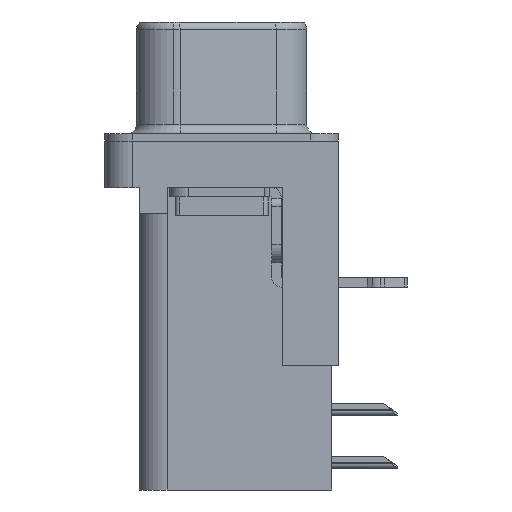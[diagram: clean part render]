
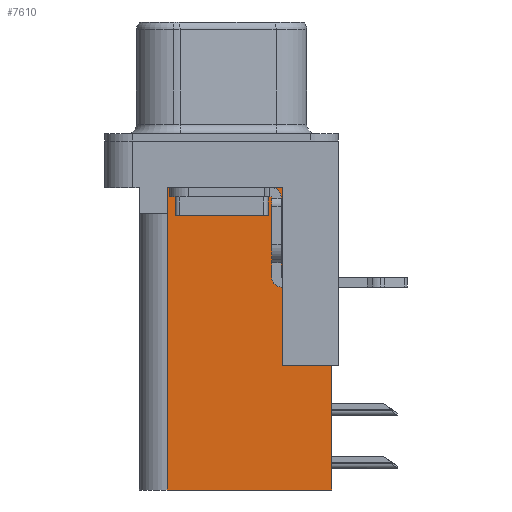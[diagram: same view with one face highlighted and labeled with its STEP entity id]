
A CAD part, left-side view. The second image highlights one B-rep face of the part: STEP entity #7610.
In plain terms, the highlighted planar face has unit normal (-1, 0, 0).
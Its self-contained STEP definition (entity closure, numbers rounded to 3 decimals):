
#11 = CARTESIAN_POINT ( 'NONE',  ( 3.7, 0., -3.9 ) ) ;
#113 = AXIS2_PLACEMENT_3D ( 'NONE', #18830, #20484, #10720 ) ;
#139 = ORIENTED_EDGE ( 'NONE', *, *, #1544, .F. ) ;
#340 = VERTEX_POINT ( 'NONE', #14604 ) ;
#858 = VECTOR ( 'NONE', #15821, 1000. ) ;
#1153 = CARTESIAN_POINT ( 'NONE',  ( 3.7, -5.925, -18.76 ) ) ;
#1157 = CARTESIAN_POINT ( 'NONE',  ( 3.7, -5.925, -2. ) ) ;
#1219 = VERTEX_POINT ( 'NONE', #19559 ) ;
#1384 = LINE ( 'NONE', #1157, #19120 ) ;
#1544 = EDGE_CURVE ( 'NONE', #19565, #340, #17263, .T. ) ;
#1650 = DIRECTION ( 'NONE',  ( 0., 1., 0. ) ) ;
#2764 = DIRECTION ( 'NONE',  ( 0., 1., 0. ) ) ;
#3130 = CARTESIAN_POINT ( 'NONE',  ( 3.7, 2.895, -3.9 ) ) ;
#3639 = VECTOR ( 'NONE', #14494, 1000. ) ;
#3640 = VECTOR ( 'NONE', #3860, 1000. ) ;
#3668 = VERTEX_POINT ( 'NONE', #13161 ) ;
#3860 = DIRECTION ( 'NONE',  ( 0., 0., -1. ) ) ;
#4145 = VECTOR ( 'NONE', #1650, 1000. ) ;
#4153 = LINE ( 'NONE', #9622, #3639 ) ;
#4337 = VECTOR ( 'NONE', #2764, 1000. ) ;
#4493 = CARTESIAN_POINT ( 'NONE',  ( 3.7, -3.295, -2.5 ) ) ;
#5072 = CARTESIAN_POINT ( 'NONE',  ( 3.7, -5.925, -12.05 ) ) ;
#5366 = VERTEX_POINT ( 'NONE', #12858 ) ;
#5698 = VECTOR ( 'NONE', #15440, 1000. ) ;
#5720 = CARTESIAN_POINT ( 'NONE',  ( 3.7, -6.295, -12.05 ) ) ;
#5996 = CARTESIAN_POINT ( 'NONE',  ( 3.7, 2.925, -3.9 ) ) ;
#6307 = CARTESIAN_POINT ( 'NONE',  ( 3.7, -3.295, -18.76 ) ) ;
#6453 = EDGE_CURVE ( 'NONE', #14682, #19565, #1384, .T. ) ;
#6469 = EDGE_CURVE ( 'NONE', #5366, #1219, #17591, .T. ) ;
#6538 = EDGE_CURVE ( 'NONE', #8450, #12078, #12741, .T. ) ;
#6655 = ORIENTED_EDGE ( 'NONE', *, *, #11893, .T. ) ;
#7006 = ORIENTED_EDGE ( 'NONE', *, *, #18163, .F. ) ;
#7356 = ORIENTED_EDGE ( 'NONE', *, *, #11287, .T. ) ;
#7496 = PLANE ( 'NONE',  #113 ) ;
#7610 = ADVANCED_FACE ( 'NONE', ( #12400 ), #7496, .F. ) ;
#8450 = VERTEX_POINT ( 'NONE', #3130 ) ;
#8936 = ORIENTED_EDGE ( 'NONE', *, *, #6538, .T. ) ;
#9622 = CARTESIAN_POINT ( 'NONE',  ( 3.7, -3.295, -18.76 ) ) ;
#9951 = ORIENTED_EDGE ( 'NONE', *, *, #6453, .F. ) ;
#9954 = ORIENTED_EDGE ( 'NONE', *, *, #6469, .T. ) ;
#10021 = LINE ( 'NONE', #5720, #5698 ) ;
#10720 = DIRECTION ( 'NONE',  ( 0., 1., 0. ) ) ;
#10790 = ORIENTED_EDGE ( 'NONE', *, *, #15153, .T. ) ;
#11287 = EDGE_CURVE ( 'NONE', #14682, #3668, #10021, .T. ) ;
#11893 = EDGE_CURVE ( 'NONE', #1219, #8450, #12241, .T. ) ;
#11927 = CARTESIAN_POINT ( 'NONE',  ( 3.7, 2.925, -18.76 ) ) ;
#12078 = VERTEX_POINT ( 'NONE', #5996 ) ;
#12241 = LINE ( 'NONE', #15208, #3640 ) ;
#12400 = FACE_OUTER_BOUND ( 'NONE', #18808, .T. ) ;
#12454 = DIRECTION ( 'NONE',  ( 0., 0., -1. ) ) ;
#12741 = LINE ( 'NONE', #11, #4145 ) ;
#12858 = CARTESIAN_POINT ( 'NONE',  ( 3.7, -3.295, -2.5 ) ) ;
#13161 = CARTESIAN_POINT ( 'NONE',  ( 3.7, -3.295, -12.05 ) ) ;
#14494 = DIRECTION ( 'NONE',  ( 0., 0., 1. ) ) ;
#14604 = CARTESIAN_POINT ( 'NONE',  ( 3.7, 2.925, -18.76 ) ) ;
#14682 = VERTEX_POINT ( 'NONE', #5072 ) ;
#15153 = EDGE_CURVE ( 'NONE', #3668, #5366, #4153, .T. ) ;
#15180 = VECTOR ( 'NONE', #16851, 1000. ) ;
#15208 = CARTESIAN_POINT ( 'NONE',  ( 3.7, 2.895, -3.9 ) ) ;
#15440 = DIRECTION ( 'NONE',  ( 0., 1., 0. ) ) ;
#15821 = DIRECTION ( 'NONE',  ( 0., 1., 0. ) ) ;
#16851 = DIRECTION ( 'NONE',  ( 0., 0., 1. ) ) ;
#17263 = LINE ( 'NONE', #6307, #4337 ) ;
#17591 = LINE ( 'NONE', #4493, #858 ) ;
#18163 = EDGE_CURVE ( 'NONE', #340, #12078, #19492, .T. ) ;
#18808 = EDGE_LOOP ( 'NONE', ( #9954, #6655, #8936, #7006, #139, #9951, #7356, #10790 ) ) ;
#18830 = CARTESIAN_POINT ( 'NONE',  ( 3.7, -3.295, -18.76 ) ) ;
#19120 = VECTOR ( 'NONE', #12454, 1000. ) ;
#19492 = LINE ( 'NONE', #11927, #15180 ) ;
#19559 = CARTESIAN_POINT ( 'NONE',  ( 3.7, 2.895, -2.5 ) ) ;
#19565 = VERTEX_POINT ( 'NONE', #1153 ) ;
#20484 = DIRECTION ( 'NONE',  ( 1., 0., 0. ) ) ;
